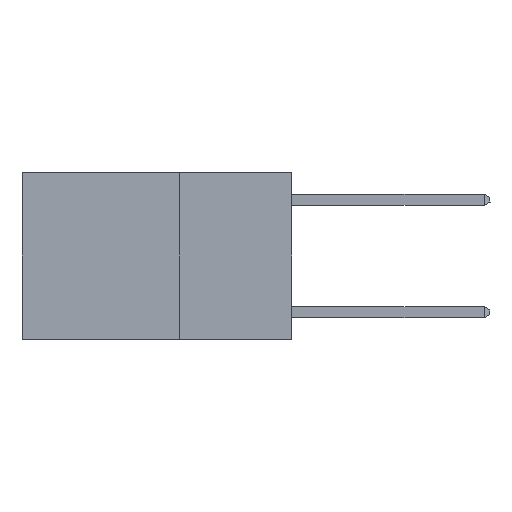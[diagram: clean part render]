
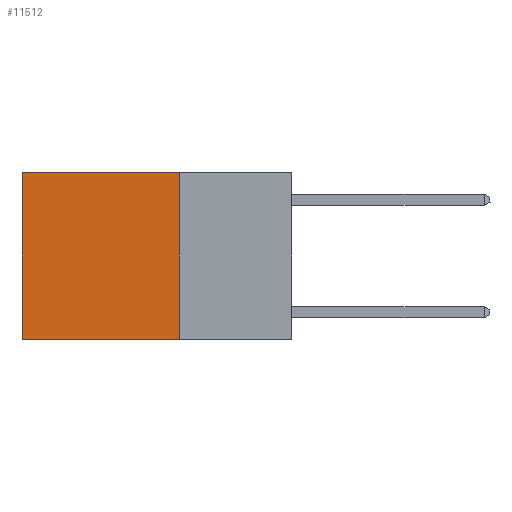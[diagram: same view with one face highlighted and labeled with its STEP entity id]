
A CAD part, left-side view. The second image highlights one B-rep face of the part: STEP entity #11512.
In plain terms, the highlighted planar face has unit normal (-1, 0, 0).
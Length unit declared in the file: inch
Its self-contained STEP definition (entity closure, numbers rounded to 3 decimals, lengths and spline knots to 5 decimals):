
#357 = CARTESIAN_POINT ( 'NONE',  ( 0.2625, 0.25, -0.37 ) ) ;
#387 = VECTOR ( 'NONE', #6674, 39.37008 ) ;
#496 = LINE ( 'NONE', #6703, #3835 ) ;
#646 = EDGE_CURVE ( 'NONE', #6226, #7094, #6809, .T. ) ;
#652 = ORIENTED_EDGE ( 'NONE', *, *, #5799, .T. ) ;
#2593 = CARTESIAN_POINT ( 'NONE',  ( 0.2625, 0.25, 0. ) ) ;
#3835 = VECTOR ( 'NONE', #18092, 39.37008 ) ;
#4600 = CARTESIAN_POINT ( 'NONE',  ( 0.2625, 0.25, 0. ) ) ;
#5042 = EDGE_CURVE ( 'NONE', #21117, #6226, #17579, .T. ) ;
#5799 = EDGE_CURVE ( 'NONE', #14464, #7094, #496, .T. ) ;
#5899 = DIRECTION ( 'NONE',  ( 0., 1., 0. ) ) ;
#6226 = VERTEX_POINT ( 'NONE', #7439 ) ;
#6674 = DIRECTION ( 'NONE',  ( 0., 1., 0. ) ) ;
#6703 = CARTESIAN_POINT ( 'NONE',  ( 0.2625, 0.6, 0. ) ) ;
#6795 = AXIS2_PLACEMENT_3D ( 'NONE', #4600, #16178, #14615 ) ;
#6809 = LINE ( 'NONE', #357, #387 ) ;
#7094 = VERTEX_POINT ( 'NONE', #15222 ) ;
#7232 = ORIENTED_EDGE ( 'NONE', *, *, #5042, .F. ) ;
#7439 = CARTESIAN_POINT ( 'NONE',  ( 0.2625, 0.25, -0.37 ) ) ;
#7569 = DIRECTION ( 'NONE',  ( 0., 0., -1. ) ) ;
#8581 = FACE_OUTER_BOUND ( 'NONE', #21074, .T. ) ;
#9581 = PLANE ( 'NONE',  #6795 ) ;
#11512 = ADVANCED_FACE ( 'NONE', ( #8581 ), #9581, .F. ) ;
#11547 = CARTESIAN_POINT ( 'NONE',  ( 0.2625, 0.6, 0. ) ) ;
#14464 = VERTEX_POINT ( 'NONE', #11547 ) ;
#14615 = DIRECTION ( 'NONE',  ( 0., 0., -1. ) ) ;
#14968 = CARTESIAN_POINT ( 'NONE',  ( 0.2625, 0.25, 0. ) ) ;
#15222 = CARTESIAN_POINT ( 'NONE',  ( 0.2625, 0.6, -0.37 ) ) ;
#16000 = EDGE_CURVE ( 'NONE', #21117, #14464, #21025, .T. ) ;
#16121 = VECTOR ( 'NONE', #5899, 39.37008 ) ;
#16178 = DIRECTION ( 'NONE',  ( 1., 0., 0. ) ) ;
#16495 = ORIENTED_EDGE ( 'NONE', *, *, #646, .F. ) ;
#17499 = CARTESIAN_POINT ( 'NONE',  ( 0.2625, 0.25, 0. ) ) ;
#17579 = LINE ( 'NONE', #17499, #17851 ) ;
#17851 = VECTOR ( 'NONE', #7569, 39.37008 ) ;
#18092 = DIRECTION ( 'NONE',  ( 0., 0., -1. ) ) ;
#18821 = ORIENTED_EDGE ( 'NONE', *, *, #16000, .T. ) ;
#21025 = LINE ( 'NONE', #2593, #16121 ) ;
#21074 = EDGE_LOOP ( 'NONE', ( #652, #16495, #7232, #18821 ) ) ;
#21117 = VERTEX_POINT ( 'NONE', #14968 ) ;
